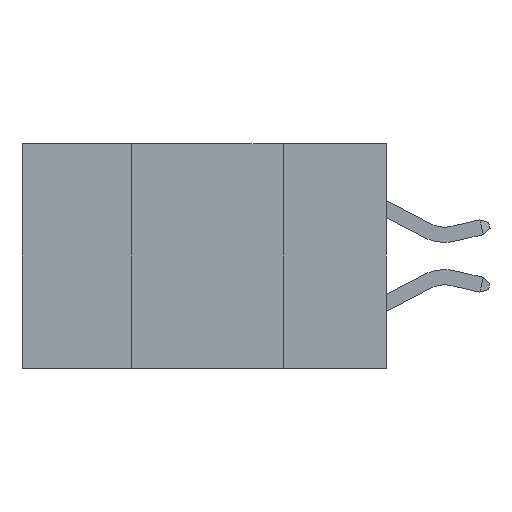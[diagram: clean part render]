
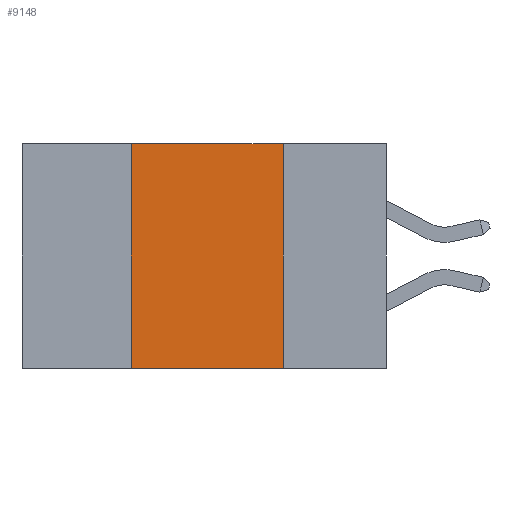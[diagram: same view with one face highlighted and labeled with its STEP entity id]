
A CAD part, left-side view. The second image highlights one B-rep face of the part: STEP entity #9148.
In plain terms, the highlighted planar face has unit normal (-1, 0, 0).
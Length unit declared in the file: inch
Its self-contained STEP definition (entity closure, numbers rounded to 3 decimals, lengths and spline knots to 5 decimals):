
#346 = VERTEX_POINT ( 'NONE', #18294 ) ;
#726 = DIRECTION ( 'NONE',  ( 0., -1., 0. ) ) ;
#1258 = DIRECTION ( 'NONE',  ( 1., 0., 0. ) ) ;
#1668 = CARTESIAN_POINT ( 'NONE',  ( 0., 0.17, -0.37 ) ) ;
#2176 = LINE ( 'NONE', #16529, #6710 ) ;
#3209 = LINE ( 'NONE', #19555, #15700 ) ;
#3904 = VECTOR ( 'NONE', #20629, 39.37008 ) ;
#3970 = CARTESIAN_POINT ( 'NONE',  ( 0., 0.17, 0. ) ) ;
#4352 = ORIENTED_EDGE ( 'NONE', *, *, #6081, .T. ) ;
#4621 = ORIENTED_EDGE ( 'NONE', *, *, #14494, .F. ) ;
#6081 = EDGE_CURVE ( 'NONE', #346, #21529, #3209, .T. ) ;
#6484 = ORIENTED_EDGE ( 'NONE', *, *, #18882, .F. ) ;
#6710 = VECTOR ( 'NONE', #11183, 39.37008 ) ;
#7937 = PLANE ( 'NONE',  #19646 ) ;
#8170 = LINE ( 'NONE', #13792, #3904 ) ;
#9148 = ADVANCED_FACE ( 'NONE', ( #12123 ), #7937, .F. ) ;
#10813 = VECTOR ( 'NONE', #12340, 39.37008 ) ;
#11183 = DIRECTION ( 'NONE',  ( 0., -1., 0. ) ) ;
#11402 = CARTESIAN_POINT ( 'NONE',  ( 0., 0.6, 0. ) ) ;
#12123 = FACE_OUTER_BOUND ( 'NONE', #15121, .T. ) ;
#12246 = CARTESIAN_POINT ( 'NONE',  ( 0., 0.17, 0. ) ) ;
#12340 = DIRECTION ( 'NONE',  ( 0., 0., -1. ) ) ;
#12812 = ORIENTED_EDGE ( 'NONE', *, *, #18904, .F. ) ;
#12997 = VERTEX_POINT ( 'NONE', #12246 ) ;
#13792 = CARTESIAN_POINT ( 'NONE',  ( 0., 0.42, 0. ) ) ;
#14494 = EDGE_CURVE ( 'NONE', #19485, #12997, #2176, .T. ) ;
#15121 = EDGE_LOOP ( 'NONE', ( #12812, #4621, #6484, #4352 ) ) ;
#15329 = LINE ( 'NONE', #3970, #10813 ) ;
#15700 = VECTOR ( 'NONE', #726, 39.37008 ) ;
#16518 = DIRECTION ( 'NONE',  ( 0., 0., -1. ) ) ;
#16529 = CARTESIAN_POINT ( 'NONE',  ( 0., 0.6, 0. ) ) ;
#18294 = CARTESIAN_POINT ( 'NONE',  ( 0., 0.42, -0.37 ) ) ;
#18882 = EDGE_CURVE ( 'NONE', #346, #19485, #8170, .T. ) ;
#18904 = EDGE_CURVE ( 'NONE', #12997, #21529, #15329, .T. ) ;
#19485 = VERTEX_POINT ( 'NONE', #19899 ) ;
#19555 = CARTESIAN_POINT ( 'NONE',  ( 0., 0.6, -0.37 ) ) ;
#19646 = AXIS2_PLACEMENT_3D ( 'NONE', #11402, #1258, #16518 ) ;
#19899 = CARTESIAN_POINT ( 'NONE',  ( 0., 0.42, 0. ) ) ;
#20629 = DIRECTION ( 'NONE',  ( 0., 0., 1. ) ) ;
#21529 = VERTEX_POINT ( 'NONE', #1668 ) ;
